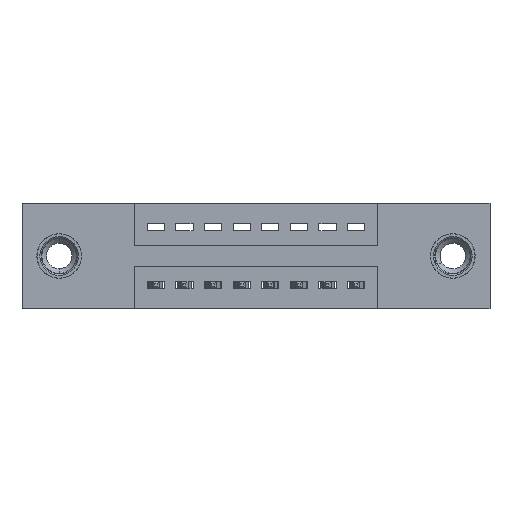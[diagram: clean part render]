
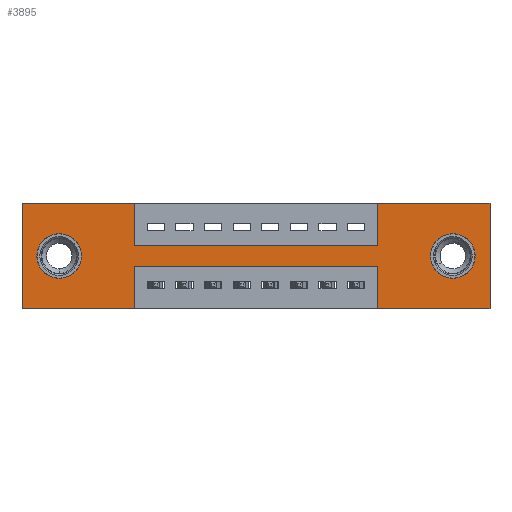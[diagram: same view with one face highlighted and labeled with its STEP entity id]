
A CAD part, front view. The second image highlights one B-rep face of the part: STEP entity #3895.
In plain terms, the highlighted planar face has unit normal (0, -1, 0).
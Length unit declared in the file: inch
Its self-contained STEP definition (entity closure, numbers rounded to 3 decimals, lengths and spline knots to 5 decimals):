
#103 = DIRECTION ( 'NONE',  ( -1., 0., 0. ) ) ;
#117 = DIRECTION ( 'NONE',  ( 0., -1., 0. ) ) ;
#308 = CIRCLE ( 'NONE', #4610, 0.078 ) ;
#363 = EDGE_CURVE ( 'NONE', #11748, #4065, #4328, .T. ) ;
#418 = LINE ( 'NONE', #4362, #10237 ) ;
#457 = CARTESIAN_POINT ( 'NONE',  ( 0.3925, 0., -0.37 ) ) ;
#542 = CARTESIAN_POINT ( 'NONE',  ( 0.13, 0., -0.185 ) ) ;
#568 = EDGE_CURVE ( 'NONE', #9389, #1959, #10322, .T. ) ;
#618 = CARTESIAN_POINT ( 'NONE',  ( 1.505, 0., -0.107 ) ) ;
#692 = ORIENTED_EDGE ( 'NONE', *, *, #1060, .F. ) ;
#830 = DIRECTION ( 'NONE',  ( -1., 0., 0. ) ) ;
#1024 = CARTESIAN_POINT ( 'NONE',  ( 0., 0., 0. ) ) ;
#1060 = EDGE_CURVE ( 'NONE', #2562, #10403, #5033, .T. ) ;
#1444 = ORIENTED_EDGE ( 'NONE', *, *, #10543, .T. ) ;
#1494 = CARTESIAN_POINT ( 'NONE',  ( 1.635, 0., 0. ) ) ;
#1548 = DIRECTION ( 'NONE',  ( 0., 0., 1. ) ) ;
#1640 = EDGE_CURVE ( 'NONE', #2732, #10669, #11590, .T. ) ;
#1774 = EDGE_CURVE ( 'NONE', #10648, #4988, #7309, .T. ) ;
#1959 = VERTEX_POINT ( 'NONE', #4586 ) ;
#2057 = CARTESIAN_POINT ( 'NONE',  ( 0.3925, 0., -0.37 ) ) ;
#2062 = CARTESIAN_POINT ( 'NONE',  ( 0., 0., -0.37 ) ) ;
#2290 = VERTEX_POINT ( 'NONE', #2057 ) ;
#2356 = ORIENTED_EDGE ( 'NONE', *, *, #568, .F. ) ;
#2375 = DIRECTION ( 'NONE',  ( 0., 1., 0. ) ) ;
#2384 = AXIS2_PLACEMENT_3D ( 'NONE', #7657, #8570, #8604 ) ;
#2444 = DIRECTION ( 'NONE',  ( 0., 0., 1. ) ) ;
#2512 = CARTESIAN_POINT ( 'NONE',  ( 0.3925, 0., -0.15 ) ) ;
#2562 = VERTEX_POINT ( 'NONE', #1494 ) ;
#2675 = LINE ( 'NONE', #9898, #11531 ) ;
#2723 = DIRECTION ( 'NONE',  ( 0., 0., -1. ) ) ;
#2732 = VERTEX_POINT ( 'NONE', #7143 ) ;
#2985 = VECTOR ( 'NONE', #5018, 39.37008 ) ;
#3002 = VECTOR ( 'NONE', #4731, 39.37008 ) ;
#3249 = EDGE_CURVE ( 'NONE', #4988, #5382, #418, .T. ) ;
#3287 = ORIENTED_EDGE ( 'NONE', *, *, #3249, .F. ) ;
#3288 = LINE ( 'NONE', #6571, #3002 ) ;
#3308 = VECTOR ( 'NONE', #6477, 39.37008 ) ;
#3344 = CARTESIAN_POINT ( 'NONE',  ( 1.2425, 0., -0.37 ) ) ;
#3357 = EDGE_CURVE ( 'NONE', #10403, #6024, #2675, .T. ) ;
#3576 = ORIENTED_EDGE ( 'NONE', *, *, #6193, .F. ) ;
#3895 = ADVANCED_FACE ( 'NONE', ( #9094, #6670, #8502 ), #11733, .T. ) ;
#4065 = VERTEX_POINT ( 'NONE', #7643 ) ;
#4081 = VERTEX_POINT ( 'NONE', #5829 ) ;
#4084 = CARTESIAN_POINT ( 'NONE',  ( 0.3925, 0., -0.15 ) ) ;
#4146 = LINE ( 'NONE', #10900, #7024 ) ;
#4328 = CIRCLE ( 'NONE', #7618, 0.078 ) ;
#4362 = CARTESIAN_POINT ( 'NONE',  ( 0., 0., 0. ) ) ;
#4369 = DIRECTION ( 'NONE',  ( 0., 1., 0. ) ) ;
#4501 = EDGE_LOOP ( 'NONE', ( #1444, #6044 ) ) ;
#4525 = EDGE_LOOP ( 'NONE', ( #9029, #4906, #3576, #5864, #692, #4894, #10510, #2356, #5736, #3287, #9825, #6704 ) ) ;
#4568 = EDGE_CURVE ( 'NONE', #2290, #10648, #4788, .T. ) ;
#4586 = CARTESIAN_POINT ( 'NONE',  ( 1.2425, 0., -0.15 ) ) ;
#4610 = AXIS2_PLACEMENT_3D ( 'NONE', #10664, #9774, #1548 ) ;
#4731 = DIRECTION ( 'NONE',  ( 0., 0., -1. ) ) ;
#4759 = LINE ( 'NONE', #5419, #9335 ) ;
#4788 = LINE ( 'NONE', #2062, #10633 ) ;
#4894 = ORIENTED_EDGE ( 'NONE', *, *, #6987, .F. ) ;
#4906 = ORIENTED_EDGE ( 'NONE', *, *, #7557, .F. ) ;
#4988 = VERTEX_POINT ( 'NONE', #7237 ) ;
#5018 = DIRECTION ( 'NONE',  ( 0., 0., -1. ) ) ;
#5033 = LINE ( 'NONE', #8062, #6050 ) ;
#5325 = DIRECTION ( 'NONE',  ( 0., 0., -1. ) ) ;
#5382 = VERTEX_POINT ( 'NONE', #9611 ) ;
#5419 = CARTESIAN_POINT ( 'NONE',  ( 1.2425, 0., -0.37 ) ) ;
#5736 = ORIENTED_EDGE ( 'NONE', *, *, #8087, .F. ) ;
#5829 = CARTESIAN_POINT ( 'NONE',  ( 1.2425, 0., -0.22 ) ) ;
#5864 = ORIENTED_EDGE ( 'NONE', *, *, #3357, .F. ) ;
#6024 = VERTEX_POINT ( 'NONE', #3344 ) ;
#6044 = ORIENTED_EDGE ( 'NONE', *, *, #1640, .T. ) ;
#6050 = VECTOR ( 'NONE', #2723, 39.37008 ) ;
#6193 = EDGE_CURVE ( 'NONE', #6024, #4081, #4759, .T. ) ;
#6251 = CARTESIAN_POINT ( 'NONE',  ( 0., 0., -0.37 ) ) ;
#6344 = AXIS2_PLACEMENT_3D ( 'NONE', #6251, #117, #11011 ) ;
#6353 = VERTEX_POINT ( 'NONE', #11127 ) ;
#6373 = DIRECTION ( 'NONE',  ( 0., 0., 1. ) ) ;
#6442 = CARTESIAN_POINT ( 'NONE',  ( 0., 0., 0. ) ) ;
#6458 = LINE ( 'NONE', #6442, #3308 ) ;
#6477 = DIRECTION ( 'NONE',  ( 1., 0., 0. ) ) ;
#6571 = CARTESIAN_POINT ( 'NONE',  ( 0.3925, 0., 0. ) ) ;
#6670 = FACE_BOUND ( 'NONE', #7390, .T. ) ;
#6699 = LINE ( 'NONE', #457, #2985 ) ;
#6704 = ORIENTED_EDGE ( 'NONE', *, *, #4568, .F. ) ;
#6987 = EDGE_CURVE ( 'NONE', #6353, #2562, #6458, .T. ) ;
#7024 = VECTOR ( 'NONE', #830, 39.37008 ) ;
#7101 = CARTESIAN_POINT ( 'NONE',  ( 0., 0., -0.37 ) ) ;
#7120 = ORIENTED_EDGE ( 'NONE', *, *, #363, .T. ) ;
#7143 = CARTESIAN_POINT ( 'NONE',  ( 1.505, 0., -0.263 ) ) ;
#7237 = CARTESIAN_POINT ( 'NONE',  ( 0., 0., 0. ) ) ;
#7309 = LINE ( 'NONE', #1024, #11025 ) ;
#7390 = EDGE_LOOP ( 'NONE', ( #7120, #11760 ) ) ;
#7557 = EDGE_CURVE ( 'NONE', #4081, #8297, #4146, .T. ) ;
#7618 = AXIS2_PLACEMENT_3D ( 'NONE', #542, #2375, #11255 ) ;
#7643 = CARTESIAN_POINT ( 'NONE',  ( 0.13, 0., -0.263 ) ) ;
#7657 = CARTESIAN_POINT ( 'NONE',  ( 1.505, 0., -0.185 ) ) ;
#7720 = AXIS2_PLACEMENT_3D ( 'NONE', #9871, #4369, #5325 ) ;
#7908 = EDGE_CURVE ( 'NONE', #4065, #11748, #308, .T. ) ;
#7953 = CARTESIAN_POINT ( 'NONE',  ( 0.13, 0., -0.107 ) ) ;
#8062 = CARTESIAN_POINT ( 'NONE',  ( 1.635, 0., 0. ) ) ;
#8087 = EDGE_CURVE ( 'NONE', #5382, #9389, #3288, .T. ) ;
#8108 = DIRECTION ( 'NONE',  ( -1., 0., 0. ) ) ;
#8181 = VECTOR ( 'NONE', #11604, 39.37008 ) ;
#8297 = VERTEX_POINT ( 'NONE', #10460 ) ;
#8401 = CARTESIAN_POINT ( 'NONE',  ( 1.635, 0., -0.37 ) ) ;
#8502 = FACE_OUTER_BOUND ( 'NONE', #4525, .T. ) ;
#8570 = DIRECTION ( 'NONE',  ( 0., 1., 0. ) ) ;
#8604 = DIRECTION ( 'NONE',  ( 0., 0., -1. ) ) ;
#8788 = EDGE_CURVE ( 'NONE', #1959, #6353, #10690, .T. ) ;
#9029 = ORIENTED_EDGE ( 'NONE', *, *, #10605, .F. ) ;
#9094 = FACE_BOUND ( 'NONE', #4501, .T. ) ;
#9128 = VECTOR ( 'NONE', #2444, 39.37008 ) ;
#9335 = VECTOR ( 'NONE', #6373, 39.37008 ) ;
#9389 = VERTEX_POINT ( 'NONE', #4084 ) ;
#9611 = CARTESIAN_POINT ( 'NONE',  ( 0.3925, 0., 0. ) ) ;
#9774 = DIRECTION ( 'NONE',  ( 0., 1., 0. ) ) ;
#9795 = CARTESIAN_POINT ( 'NONE',  ( 1.2425, 0., 0. ) ) ;
#9825 = ORIENTED_EDGE ( 'NONE', *, *, #1774, .F. ) ;
#9871 = CARTESIAN_POINT ( 'NONE',  ( 1.505, 0., -0.185 ) ) ;
#9898 = CARTESIAN_POINT ( 'NONE',  ( 0., 0., -0.37 ) ) ;
#10237 = VECTOR ( 'NONE', #10713, 39.37008 ) ;
#10322 = LINE ( 'NONE', #2512, #8181 ) ;
#10392 = CIRCLE ( 'NONE', #2384, 0.078 ) ;
#10403 = VERTEX_POINT ( 'NONE', #8401 ) ;
#10460 = CARTESIAN_POINT ( 'NONE',  ( 0.3925, 0., -0.22 ) ) ;
#10510 = ORIENTED_EDGE ( 'NONE', *, *, #8788, .F. ) ;
#10543 = EDGE_CURVE ( 'NONE', #10669, #2732, #10392, .T. ) ;
#10605 = EDGE_CURVE ( 'NONE', #8297, #2290, #6699, .T. ) ;
#10633 = VECTOR ( 'NONE', #103, 39.37008 ) ;
#10648 = VERTEX_POINT ( 'NONE', #7101 ) ;
#10664 = CARTESIAN_POINT ( 'NONE',  ( 0.13, 0., -0.185 ) ) ;
#10669 = VERTEX_POINT ( 'NONE', #618 ) ;
#10690 = LINE ( 'NONE', #9795, #9128 ) ;
#10713 = DIRECTION ( 'NONE',  ( 1., 0., 0. ) ) ;
#10900 = CARTESIAN_POINT ( 'NONE',  ( 0.3925, 0., -0.22 ) ) ;
#11011 = DIRECTION ( 'NONE',  ( 0., 0., -1. ) ) ;
#11025 = VECTOR ( 'NONE', #11056, 39.37008 ) ;
#11056 = DIRECTION ( 'NONE',  ( 0., 0., 1. ) ) ;
#11127 = CARTESIAN_POINT ( 'NONE',  ( 1.2425, 0., 0. ) ) ;
#11255 = DIRECTION ( 'NONE',  ( 0., 0., 1. ) ) ;
#11531 = VECTOR ( 'NONE', #8108, 39.37008 ) ;
#11590 = CIRCLE ( 'NONE', #7720, 0.078 ) ;
#11604 = DIRECTION ( 'NONE',  ( 1., 0., 0. ) ) ;
#11733 = PLANE ( 'NONE',  #6344 ) ;
#11748 = VERTEX_POINT ( 'NONE', #7953 ) ;
#11760 = ORIENTED_EDGE ( 'NONE', *, *, #7908, .T. ) ;
